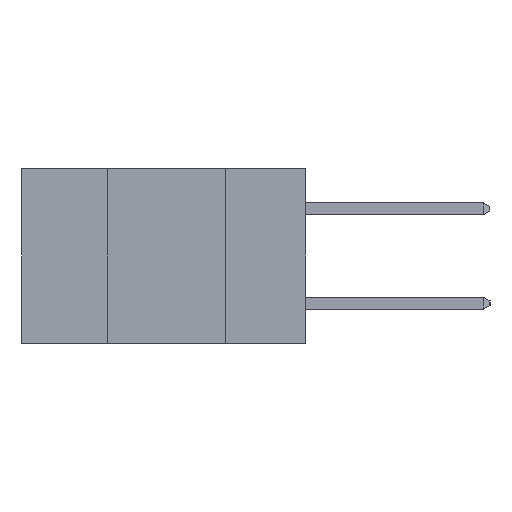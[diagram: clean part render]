
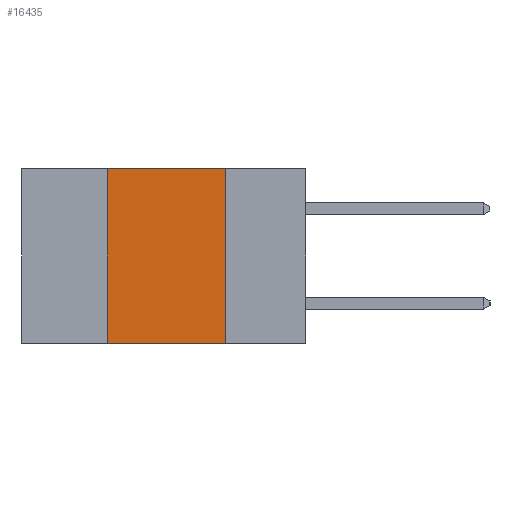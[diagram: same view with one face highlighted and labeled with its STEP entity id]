
A CAD part, left-side view. The second image highlights one B-rep face of the part: STEP entity #16435.
In plain terms, the highlighted planar face has unit normal (-1, 0, 0).
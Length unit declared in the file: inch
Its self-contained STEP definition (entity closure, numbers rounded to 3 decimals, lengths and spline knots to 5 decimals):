
#1102 = CARTESIAN_POINT ( 'NONE',  ( 0., 0.42, -0.37 ) ) ;
#1231 = EDGE_CURVE ( 'NONE', #4440, #5505, #3812, .T. ) ;
#1537 = VECTOR ( 'NONE', #15218, 39.37008 ) ;
#1575 = CARTESIAN_POINT ( 'NONE',  ( 0., 0.6, 0. ) ) ;
#2112 = VECTOR ( 'NONE', #5136, 39.37008 ) ;
#2280 = DIRECTION ( 'NONE',  ( 1., 0., 0. ) ) ;
#3812 = LINE ( 'NONE', #1575, #7766 ) ;
#3865 = ORIENTED_EDGE ( 'NONE', *, *, #13813, .F. ) ;
#4332 = EDGE_CURVE ( 'NONE', #9462, #4440, #8756, .T. ) ;
#4440 = VERTEX_POINT ( 'NONE', #12222 ) ;
#4963 = CARTESIAN_POINT ( 'NONE',  ( 0., 0.6, 0. ) ) ;
#5136 = DIRECTION ( 'NONE',  ( 0., -1., 0. ) ) ;
#5327 = ORIENTED_EDGE ( 'NONE', *, *, #1231, .F. ) ;
#5505 = VERTEX_POINT ( 'NONE', #14442 ) ;
#6361 = FACE_OUTER_BOUND ( 'NONE', #14947, .T. ) ;
#7766 = VECTOR ( 'NONE', #8423, 39.37008 ) ;
#7790 = CARTESIAN_POINT ( 'NONE',  ( 0., 0.6, -0.37 ) ) ;
#7885 = CARTESIAN_POINT ( 'NONE',  ( 0., 0.42, -0.37 ) ) ;
#8423 = DIRECTION ( 'NONE',  ( 0., -1., 0. ) ) ;
#8756 = LINE ( 'NONE', #1102, #1537 ) ;
#9002 = PLANE ( 'NONE',  #10056 ) ;
#9462 = VERTEX_POINT ( 'NONE', #7885 ) ;
#9710 = LINE ( 'NONE', #9989, #15823 ) ;
#9736 = LINE ( 'NONE', #7790, #2112 ) ;
#9989 = CARTESIAN_POINT ( 'NONE',  ( 0., 0.17, -0.37 ) ) ;
#10056 = AXIS2_PLACEMENT_3D ( 'NONE', #4963, #2280, #11716 ) ;
#11328 = DIRECTION ( 'NONE',  ( 0., 0., -1. ) ) ;
#11716 = DIRECTION ( 'NONE',  ( 0., 0., -1. ) ) ;
#11967 = CARTESIAN_POINT ( 'NONE',  ( 0., 0.17, -0.37 ) ) ;
#12222 = CARTESIAN_POINT ( 'NONE',  ( 0., 0.42, 0. ) ) ;
#12943 = EDGE_CURVE ( 'NONE', #9462, #13016, #9736, .T. ) ;
#13016 = VERTEX_POINT ( 'NONE', #11967 ) ;
#13813 = EDGE_CURVE ( 'NONE', #5505, #13016, #9710, .T. ) ;
#14442 = CARTESIAN_POINT ( 'NONE',  ( 0., 0.17, 0. ) ) ;
#14947 = EDGE_LOOP ( 'NONE', ( #3865, #5327, #15439, #15039 ) ) ;
#15039 = ORIENTED_EDGE ( 'NONE', *, *, #12943, .T. ) ;
#15218 = DIRECTION ( 'NONE',  ( 0., 0., 1. ) ) ;
#15439 = ORIENTED_EDGE ( 'NONE', *, *, #4332, .F. ) ;
#15823 = VECTOR ( 'NONE', #11328, 39.37008 ) ;
#16435 = ADVANCED_FACE ( 'NONE', ( #6361 ), #9002, .F. ) ;
